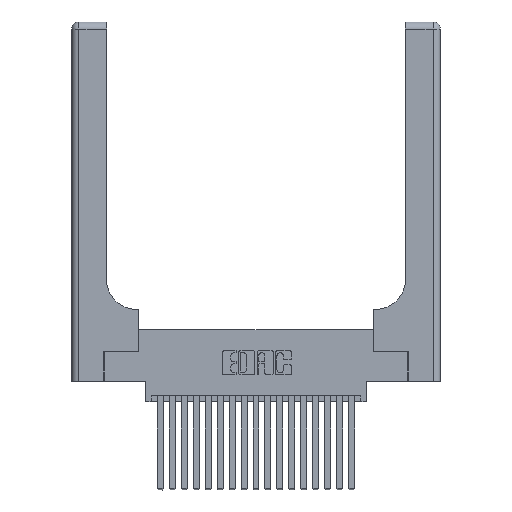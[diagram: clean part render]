
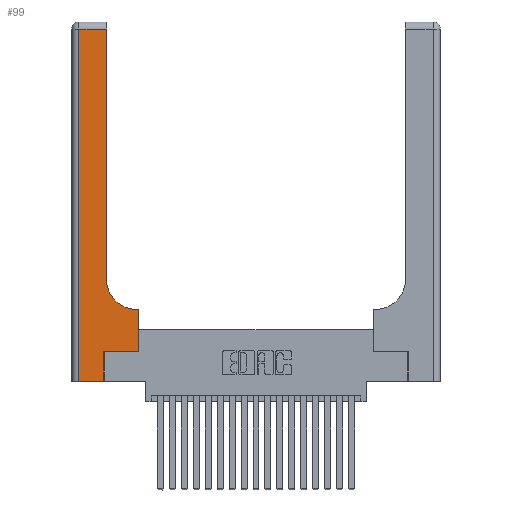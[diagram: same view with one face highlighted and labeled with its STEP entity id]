
A CAD part, top view. The second image highlights one B-rep face of the part: STEP entity #99.
In plain terms, the highlighted planar face has unit normal (0, 0, 1).
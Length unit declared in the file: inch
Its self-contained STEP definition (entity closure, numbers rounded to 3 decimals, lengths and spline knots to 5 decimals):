
#99 = ADVANCED_FACE ( 'NONE', ( #9733 ), #8641, .F. ) ;
#254 = VERTEX_POINT ( 'NONE', #15126 ) ;
#594 = CARTESIAN_POINT ( 'NONE',  ( 0.269, 0., 0.37 ) ) ;
#643 = ORIENTED_EDGE ( 'NONE', *, *, #7568, .T. ) ;
#1123 = LINE ( 'NONE', #4487, #6161 ) ;
#1140 = EDGE_CURVE ( 'NONE', #8568, #5833, #19546, .T. ) ;
#1416 = VERTEX_POINT ( 'NONE', #7743 ) ;
#1493 = CARTESIAN_POINT ( 'NONE',  ( 0.5415, 0.85, 0.37 ) ) ;
#2043 = CARTESIAN_POINT ( 'NONE',  ( 0., 3., 0.37 ) ) ;
#2685 = LINE ( 'NONE', #594, #20877 ) ;
#2945 = LINE ( 'NONE', #14202, #20349 ) ;
#3112 = VECTOR ( 'NONE', #16864, 39.37008 ) ;
#3149 = ORIENTED_EDGE ( 'NONE', *, *, #11649, .T. ) ;
#3618 = ORIENTED_EDGE ( 'NONE', *, *, #9594, .T. ) ;
#3969 = VECTOR ( 'NONE', #13281, 39.37008 ) ;
#4047 = DIRECTION ( 'NONE',  ( -1., 0., 0. ) ) ;
#4487 = CARTESIAN_POINT ( 'NONE',  ( 0.269, 0.25, 0.37 ) ) ;
#4518 = LINE ( 'NONE', #6772, #3969 ) ;
#4782 = ORIENTED_EDGE ( 'NONE', *, *, #9428, .T. ) ;
#5221 = CARTESIAN_POINT ( 'NONE',  ( 0., 0., 0.37 ) ) ;
#5298 = CARTESIAN_POINT ( 'NONE',  ( 0.06, 3., 0.37 ) ) ;
#5344 = DIRECTION ( 'NONE',  ( 0., 1., 0. ) ) ;
#5622 = ORIENTED_EDGE ( 'NONE', *, *, #1140, .T. ) ;
#5731 = VERTEX_POINT ( 'NONE', #20568 ) ;
#5833 = VERTEX_POINT ( 'NONE', #10629 ) ;
#6126 = CARTESIAN_POINT ( 'NONE',  ( 0.5585, 0.25, 0.37 ) ) ;
#6161 = VECTOR ( 'NONE', #8010, 39.37008 ) ;
#6668 = AXIS2_PLACEMENT_3D ( 'NONE', #1493, #10062, #21690 ) ;
#6772 = CARTESIAN_POINT ( 'NONE',  ( 0.2915, 0.6, 0.37 ) ) ;
#6872 = CARTESIAN_POINT ( 'NONE',  ( 0.2915, 2.94, 0.37 ) ) ;
#7009 = ORIENTED_EDGE ( 'NONE', *, *, #18769, .T. ) ;
#7273 = EDGE_CURVE ( 'NONE', #8584, #254, #2685, .T. ) ;
#7372 = ORIENTED_EDGE ( 'NONE', *, *, #15449, .T. ) ;
#7568 = EDGE_CURVE ( 'NONE', #9170, #17730, #14820, .T. ) ;
#7712 = LINE ( 'NONE', #15417, #15591 ) ;
#7743 = CARTESIAN_POINT ( 'NONE',  ( 0.06, 2.94, 0.37 ) ) ;
#8010 = DIRECTION ( 'NONE',  ( 1., 0., 0. ) ) ;
#8568 = VERTEX_POINT ( 'NONE', #14692 ) ;
#8584 = VERTEX_POINT ( 'NONE', #16310 ) ;
#8641 = PLANE ( 'NONE',  #12044 ) ;
#8664 = LINE ( 'NONE', #5298, #3112 ) ;
#8769 = VECTOR ( 'NONE', #12162, 39.37008 ) ;
#9170 = VERTEX_POINT ( 'NONE', #6126 ) ;
#9428 = EDGE_CURVE ( 'NONE', #5731, #8584, #10079, .T. ) ;
#9594 = EDGE_CURVE ( 'NONE', #11186, #1416, #2945, .T. ) ;
#9733 = FACE_OUTER_BOUND ( 'NONE', #17733, .T. ) ;
#9901 = EDGE_CURVE ( 'NONE', #5833, #11186, #7712, .T. ) ;
#10062 = DIRECTION ( 'NONE',  ( 0., 0., -1. ) ) ;
#10079 = LINE ( 'NONE', #5221, #8769 ) ;
#10181 = ORIENTED_EDGE ( 'NONE', *, *, #7273, .T. ) ;
#10322 = DIRECTION ( 'NONE',  ( 0., 1., 0. ) ) ;
#10629 = CARTESIAN_POINT ( 'NONE',  ( 0.2915, 0.85, 0.37 ) ) ;
#11186 = VERTEX_POINT ( 'NONE', #6872 ) ;
#11649 = EDGE_CURVE ( 'NONE', #17730, #8568, #4518, .T. ) ;
#12044 = AXIS2_PLACEMENT_3D ( 'NONE', #2043, #20420, #13739 ) ;
#12162 = DIRECTION ( 'NONE',  ( 1., 0., 0. ) ) ;
#12894 = ORIENTED_EDGE ( 'NONE', *, *, #9901, .T. ) ;
#13281 = DIRECTION ( 'NONE',  ( -1., 0., 0. ) ) ;
#13665 = CARTESIAN_POINT ( 'NONE',  ( 0.5585, 0.25, 0.37 ) ) ;
#13739 = DIRECTION ( 'NONE',  ( -1., 0., 0. ) ) ;
#13900 = DIRECTION ( 'NONE',  ( 0., 1., 0. ) ) ;
#14010 = VECTOR ( 'NONE', #10322, 39.37008 ) ;
#14202 = CARTESIAN_POINT ( 'NONE',  ( 0., 2.94, 0.37 ) ) ;
#14692 = CARTESIAN_POINT ( 'NONE',  ( 0.5415, 0.6, 0.37 ) ) ;
#14820 = LINE ( 'NONE', #13665, #14010 ) ;
#15126 = CARTESIAN_POINT ( 'NONE',  ( 0.269, 0.25, 0.37 ) ) ;
#15417 = CARTESIAN_POINT ( 'NONE',  ( 0.2915, 3., 0.37 ) ) ;
#15449 = EDGE_CURVE ( 'NONE', #254, #9170, #1123, .T. ) ;
#15591 = VECTOR ( 'NONE', #5344, 39.37008 ) ;
#16310 = CARTESIAN_POINT ( 'NONE',  ( 0.269, 0., 0.37 ) ) ;
#16864 = DIRECTION ( 'NONE',  ( 0., -1., 0. ) ) ;
#17730 = VERTEX_POINT ( 'NONE', #20962 ) ;
#17733 = EDGE_LOOP ( 'NONE', ( #12894, #3618, #7009, #4782, #10181, #7372, #643, #3149, #5622 ) ) ;
#18769 = EDGE_CURVE ( 'NONE', #1416, #5731, #8664, .T. ) ;
#19546 = CIRCLE ( 'NONE', #6668, 0.25 ) ;
#20349 = VECTOR ( 'NONE', #4047, 39.37008 ) ;
#20420 = DIRECTION ( 'NONE',  ( 0., 0., -1. ) ) ;
#20568 = CARTESIAN_POINT ( 'NONE',  ( 0.06, 0., 0.37 ) ) ;
#20877 = VECTOR ( 'NONE', #13900, 39.37008 ) ;
#20962 = CARTESIAN_POINT ( 'NONE',  ( 0.5585, 0.6, 0.37 ) ) ;
#21690 = DIRECTION ( 'NONE',  ( 1., 0., 0. ) ) ;
